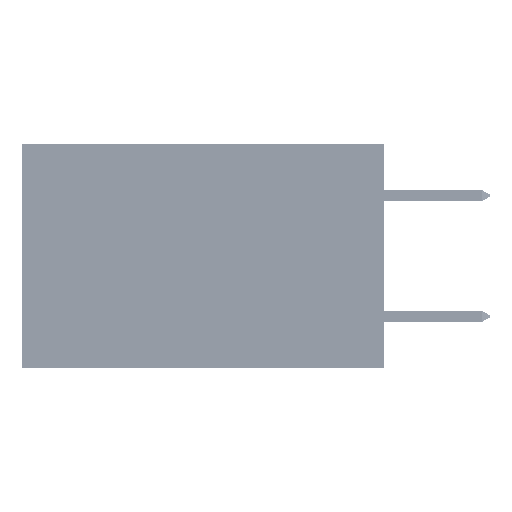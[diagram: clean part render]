
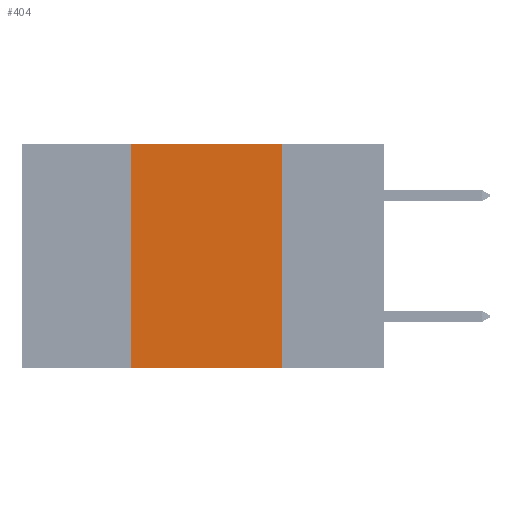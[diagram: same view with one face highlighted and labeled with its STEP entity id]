
A CAD part, left-side view. The second image highlights one B-rep face of the part: STEP entity #404.
In plain terms, the highlighted planar face has unit normal (-1, 0, 0).
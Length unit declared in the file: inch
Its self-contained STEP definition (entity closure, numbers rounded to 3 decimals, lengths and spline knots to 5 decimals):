
#240 = CARTESIAN_POINT ( 'NONE',  ( 0., 0.42, -0.37 ) ) ;
#404 = ADVANCED_FACE ( 'NONE', ( #38935 ), #14899, .F. ) ;
#1876 = CARTESIAN_POINT ( 'NONE',  ( 0., 0.6, -0.37 ) ) ;
#2787 = CARTESIAN_POINT ( 'NONE',  ( 0., 0.17, -0.37 ) ) ;
#2977 = EDGE_CURVE ( 'NONE', #7933, #14368, #8311, .T. ) ;
#4879 = VECTOR ( 'NONE', #27310, 39.37008 ) ;
#7228 = CARTESIAN_POINT ( 'NONE',  ( 0., 0.42, 0. ) ) ;
#7933 = VERTEX_POINT ( 'NONE', #240 ) ;
#8311 = LINE ( 'NONE', #36516, #45657 ) ;
#8425 = LINE ( 'NONE', #31387, #16398 ) ;
#10109 = DIRECTION ( 'NONE',  ( 0., 0., -1. ) ) ;
#14368 = VERTEX_POINT ( 'NONE', #7228 ) ;
#14718 = ORIENTED_EDGE ( 'NONE', *, *, #32734, .F. ) ;
#14899 = PLANE ( 'NONE',  #34565 ) ;
#16398 = VECTOR ( 'NONE', #28995, 39.37008 ) ;
#17019 = EDGE_LOOP ( 'NONE', ( #33432, #14718, #28520, #33862 ) ) ;
#18083 = EDGE_CURVE ( 'NONE', #7933, #20078, #41197, .T. ) ;
#20078 = VERTEX_POINT ( 'NONE', #2787 ) ;
#24857 = CARTESIAN_POINT ( 'NONE',  ( 0., 0.6, 0. ) ) ;
#25928 = VERTEX_POINT ( 'NONE', #42919 ) ;
#27310 = DIRECTION ( 'NONE',  ( 0., -1., 0. ) ) ;
#28520 = ORIENTED_EDGE ( 'NONE', *, *, #2977, .F. ) ;
#28995 = DIRECTION ( 'NONE',  ( 0., -1., 0. ) ) ;
#31387 = CARTESIAN_POINT ( 'NONE',  ( 0., 0.6, 0. ) ) ;
#32734 = EDGE_CURVE ( 'NONE', #14368, #25928, #8425, .T. ) ;
#33385 = EDGE_CURVE ( 'NONE', #25928, #20078, #38986, .T. ) ;
#33432 = ORIENTED_EDGE ( 'NONE', *, *, #33385, .F. ) ;
#33862 = ORIENTED_EDGE ( 'NONE', *, *, #18083, .T. ) ;
#34565 = AXIS2_PLACEMENT_3D ( 'NONE', #24857, #38242, #39698 ) ;
#36150 = VECTOR ( 'NONE', #10109, 39.37008 ) ;
#36516 = CARTESIAN_POINT ( 'NONE',  ( 0., 0.42, 0. ) ) ;
#37154 = DIRECTION ( 'NONE',  ( 0., 0., 1. ) ) ;
#38242 = DIRECTION ( 'NONE',  ( 1., 0., 0. ) ) ;
#38935 = FACE_OUTER_BOUND ( 'NONE', #17019, .T. ) ;
#38941 = CARTESIAN_POINT ( 'NONE',  ( 0., 0.17, 0. ) ) ;
#38986 = LINE ( 'NONE', #38941, #36150 ) ;
#39698 = DIRECTION ( 'NONE',  ( 0., 0., -1. ) ) ;
#41197 = LINE ( 'NONE', #1876, #4879 ) ;
#42919 = CARTESIAN_POINT ( 'NONE',  ( 0., 0.17, 0. ) ) ;
#45657 = VECTOR ( 'NONE', #37154, 39.37008 ) ;
